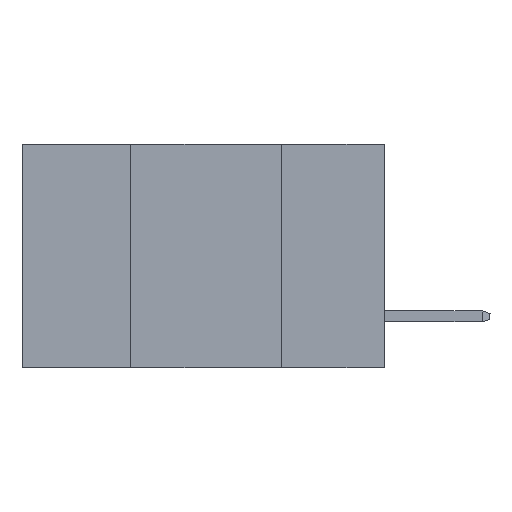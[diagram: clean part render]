
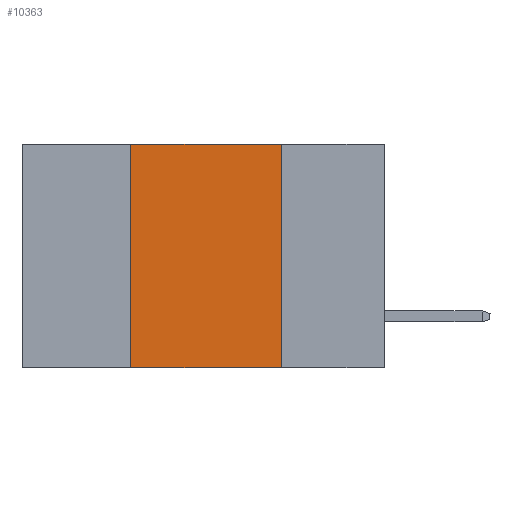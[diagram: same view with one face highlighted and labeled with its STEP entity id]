
A CAD part, left-side view. The second image highlights one B-rep face of the part: STEP entity #10363.
In plain terms, the highlighted planar face has unit normal (-1, 0, 0).
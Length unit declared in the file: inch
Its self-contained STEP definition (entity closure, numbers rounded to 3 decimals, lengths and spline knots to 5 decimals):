
#48 = DIRECTION ( 'NONE',  ( 0., 0., 1. ) ) ;
#243 = VECTOR ( 'NONE', #48, 39.37008 ) ;
#1489 = VECTOR ( 'NONE', #23463, 39.37008 ) ;
#1938 = EDGE_LOOP ( 'NONE', ( #11414, #2000, #5289, #13676 ) ) ;
#1996 = CARTESIAN_POINT ( 'NONE',  ( 0., 0.42, 0. ) ) ;
#2000 = ORIENTED_EDGE ( 'NONE', *, *, #15764, .F. ) ;
#2913 = VERTEX_POINT ( 'NONE', #13962 ) ;
#3217 = DIRECTION ( 'NONE',  ( 0., 0., -1. ) ) ;
#3245 = DIRECTION ( 'NONE',  ( 1., 0., 0. ) ) ;
#3271 = PLANE ( 'NONE',  #9037 ) ;
#3390 = CARTESIAN_POINT ( 'NONE',  ( 0., 0.6, 0. ) ) ;
#3422 = LINE ( 'NONE', #19201, #17389 ) ;
#4265 = DIRECTION ( 'NONE',  ( 0., 0., -1. ) ) ;
#4587 = CARTESIAN_POINT ( 'NONE',  ( 0., 0.17, -0.37 ) ) ;
#4722 = EDGE_CURVE ( 'NONE', #2913, #21395, #7298, .T. ) ;
#5289 = ORIENTED_EDGE ( 'NONE', *, *, #12220, .F. ) ;
#7298 = LINE ( 'NONE', #4587, #11047 ) ;
#7470 = CARTESIAN_POINT ( 'NONE',  ( 0., 0.6, -0.37 ) ) ;
#8203 = EDGE_CURVE ( 'NONE', #14981, #21395, #10914, .T. ) ;
#9037 = AXIS2_PLACEMENT_3D ( 'NONE', #3390, #3245, #3217 ) ;
#9851 = CARTESIAN_POINT ( 'NONE',  ( 0., 0.17, -0.37 ) ) ;
#10363 = ADVANCED_FACE ( 'NONE', ( #22829 ), #3271, .F. ) ;
#10914 = LINE ( 'NONE', #7470, #1489 ) ;
#11047 = VECTOR ( 'NONE', #4265, 39.37008 ) ;
#11414 = ORIENTED_EDGE ( 'NONE', *, *, #4722, .F. ) ;
#11455 = CARTESIAN_POINT ( 'NONE',  ( 0., 0.42, -0.37 ) ) ;
#12220 = EDGE_CURVE ( 'NONE', #14981, #14207, #18618, .T. ) ;
#13676 = ORIENTED_EDGE ( 'NONE', *, *, #8203, .T. ) ;
#13962 = CARTESIAN_POINT ( 'NONE',  ( 0., 0.17, 0. ) ) ;
#14124 = DIRECTION ( 'NONE',  ( 0., -1., 0. ) ) ;
#14207 = VERTEX_POINT ( 'NONE', #1996 ) ;
#14981 = VERTEX_POINT ( 'NONE', #15030 ) ;
#15030 = CARTESIAN_POINT ( 'NONE',  ( 0., 0.42, -0.37 ) ) ;
#15764 = EDGE_CURVE ( 'NONE', #14207, #2913, #3422, .T. ) ;
#17389 = VECTOR ( 'NONE', #14124, 39.37008 ) ;
#18618 = LINE ( 'NONE', #11455, #243 ) ;
#19201 = CARTESIAN_POINT ( 'NONE',  ( 0., 0.6, 0. ) ) ;
#21395 = VERTEX_POINT ( 'NONE', #9851 ) ;
#22829 = FACE_OUTER_BOUND ( 'NONE', #1938, .T. ) ;
#23463 = DIRECTION ( 'NONE',  ( 0., -1., 0. ) ) ;
